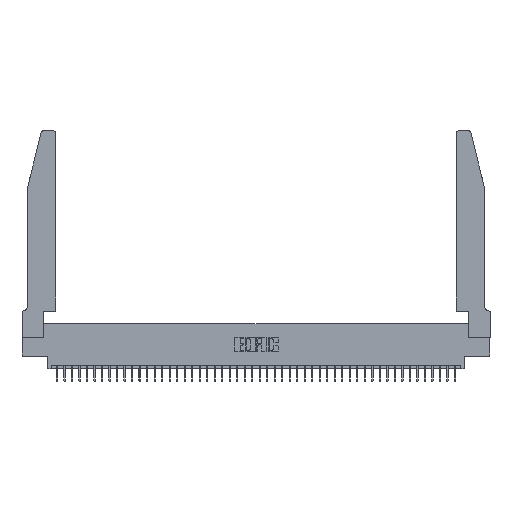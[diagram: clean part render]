
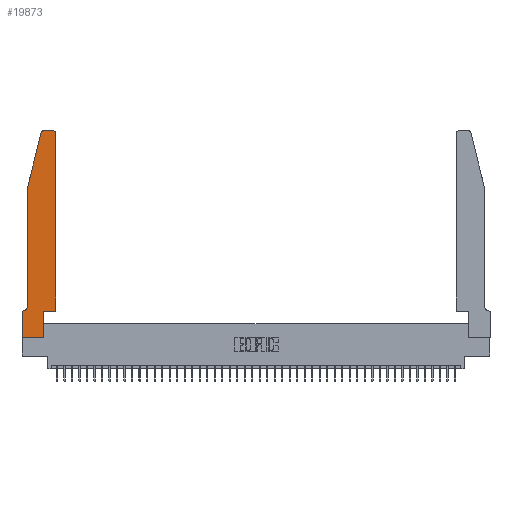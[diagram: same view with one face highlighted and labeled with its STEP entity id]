
A CAD part, top view. The second image highlights one B-rep face of the part: STEP entity #19873.
In plain terms, the highlighted planar face has unit normal (0, 0, 1).
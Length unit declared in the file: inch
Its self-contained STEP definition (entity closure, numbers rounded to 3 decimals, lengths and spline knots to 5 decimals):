
#1806 = CIRCLE ( 'NONE', #24319, 0.03 ) ;
#1857 = ORIENTED_EDGE ( 'NONE', *, *, #44088, .T. ) ;
#3058 = DIRECTION ( 'NONE',  ( 0., 1., 0. ) ) ;
#3879 = EDGE_CURVE ( 'NONE', #10807, #8634, #20952, .T. ) ;
#3942 = VERTEX_POINT ( 'NONE', #7230 ) ;
#4256 = ORIENTED_EDGE ( 'NONE', *, *, #16761, .T. ) ;
#4338 = DIRECTION ( 'NONE',  ( 0., 1., 0. ) ) ;
#4415 = AXIS2_PLACEMENT_3D ( 'NONE', #12191, #8808, #37184 ) ;
#4434 = CARTESIAN_POINT ( 'NONE',  ( 0.0755, 0.35, 0.37 ) ) ;
#4699 = EDGE_CURVE ( 'NONE', #20793, #45562, #8791, .T. ) ;
#4736 = CARTESIAN_POINT ( 'NONE',  ( 0., 0.35, 0.37 ) ) ;
#5658 = CARTESIAN_POINT ( 'NONE',  ( 0.0055, 0.42, 0.37 ) ) ;
#5793 = DIRECTION ( 'NONE',  ( 1., 0., 0. ) ) ;
#5996 = CARTESIAN_POINT ( 'NONE',  ( 0.2865, 0., 0.37 ) ) ;
#7230 = CARTESIAN_POINT ( 'NONE',  ( 0.284, 2.75, 0.37 ) ) ;
#7281 = LINE ( 'NONE', #4434, #15554 ) ;
#7769 = DIRECTION ( 'NONE',  ( 0., -1., 0. ) ) ;
#7910 = CARTESIAN_POINT ( 'NONE',  ( 0., 0., 0.37 ) ) ;
#8146 = ORIENTED_EDGE ( 'NONE', *, *, #43980, .T. ) ;
#8273 = DIRECTION ( 'NONE',  ( 1., 0., 0. ) ) ;
#8634 = VERTEX_POINT ( 'NONE', #21902 ) ;
#8762 = ORIENTED_EDGE ( 'NONE', *, *, #3879, .T. ) ;
#8791 = LINE ( 'NONE', #39439, #13723 ) ;
#8808 = DIRECTION ( 'NONE',  ( 0., 0., 1. ) ) ;
#9074 = CARTESIAN_POINT ( 'NONE',  ( 0., 0.35, 0.37 ) ) ;
#9474 = CIRCLE ( 'NONE', #20605, 0.07 ) ;
#10147 = ORIENTED_EDGE ( 'NONE', *, *, #39476, .T. ) ;
#10807 = VERTEX_POINT ( 'NONE', #34478 ) ;
#11122 = VECTOR ( 'NONE', #7769, 39.37008 ) ;
#11125 = EDGE_CURVE ( 'NONE', #25352, #10807, #15219, .T. ) ;
#11546 = DIRECTION ( 'NONE',  ( -1., 0., 0. ) ) ;
#11575 = LINE ( 'NONE', #18360, #22046 ) ;
#11656 = EDGE_LOOP ( 'NONE', ( #17000, #4256, #24188, #25541, #1857, #8146, #19244, #37994, #45067, #42346, #8762, #10147 ) ) ;
#12086 = DIRECTION ( 'NONE',  ( -1., 0., 0. ) ) ;
#12191 = CARTESIAN_POINT ( 'NONE',  ( 0.284, 2.72, 0.37 ) ) ;
#12465 = EDGE_CURVE ( 'NONE', #45123, #3942, #37187, .T. ) ;
#12601 = DIRECTION ( 'NONE',  ( 0., 0., 1. ) ) ;
#13723 = VECTOR ( 'NONE', #32603, 39.37008 ) ;
#13988 = LINE ( 'NONE', #44260, #25604 ) ;
#14217 = CARTESIAN_POINT ( 'NONE',  ( 0.4205, 2.75, 0.37 ) ) ;
#14949 = VECTOR ( 'NONE', #4338, 39.37008 ) ;
#15026 = CARTESIAN_POINT ( 'NONE',  ( 0.4505, 0.35, 0.37 ) ) ;
#15204 = DIRECTION ( 'NONE',  ( 0., 0., 1. ) ) ;
#15219 = LINE ( 'NONE', #15026, #20151 ) ;
#15293 = VERTEX_POINT ( 'NONE', #4736 ) ;
#15458 = EDGE_CURVE ( 'NONE', #15293, #20793, #13988, .T. ) ;
#15504 = AXIS2_PLACEMENT_3D ( 'NONE', #9074, #12601, #5793 ) ;
#15554 = VECTOR ( 'NONE', #11546, 39.37008 ) ;
#16761 = EDGE_CURVE ( 'NONE', #3942, #23194, #39832, .T. ) ;
#17000 = ORIENTED_EDGE ( 'NONE', *, *, #12465, .T. ) ;
#18360 = CARTESIAN_POINT ( 'NONE',  ( 0.0755, 2., 0.37 ) ) ;
#19244 = ORIENTED_EDGE ( 'NONE', *, *, #15458, .T. ) ;
#19538 = DIRECTION ( 'NONE',  ( 0., 0., -1. ) ) ;
#19554 = VERTEX_POINT ( 'NONE', #22153 ) ;
#19873 = ADVANCED_FACE ( 'NONE', ( #30736 ), #26960, .T. ) ;
#20133 = DIRECTION ( 'NONE',  ( 0., -1., 0. ) ) ;
#20151 = VECTOR ( 'NONE', #36160, 39.37008 ) ;
#20487 = CARTESIAN_POINT ( 'NONE',  ( 0.4505, 0.35, 0.37 ) ) ;
#20605 = AXIS2_PLACEMENT_3D ( 'NONE', #5658, #19538, #34046 ) ;
#20793 = VERTEX_POINT ( 'NONE', #7910 ) ;
#20952 = LINE ( 'NONE', #20487, #39786 ) ;
#21011 = CARTESIAN_POINT ( 'NONE',  ( 0.0755, 2., 0.37 ) ) ;
#21902 = CARTESIAN_POINT ( 'NONE',  ( 0.4505, 2.72, 0.37 ) ) ;
#22046 = VECTOR ( 'NONE', #43245, 39.37008 ) ;
#22153 = CARTESIAN_POINT ( 'NONE',  ( 0.0755, 0.42, 0.37 ) ) ;
#23194 = VERTEX_POINT ( 'NONE', #42938 ) ;
#24188 = ORIENTED_EDGE ( 'NONE', *, *, #45297, .T. ) ;
#24250 = VERTEX_POINT ( 'NONE', #21011 ) ;
#24319 = AXIS2_PLACEMENT_3D ( 'NONE', #25851, #15204, #8273 ) ;
#25352 = VERTEX_POINT ( 'NONE', #37000 ) ;
#25541 = ORIENTED_EDGE ( 'NONE', *, *, #43533, .T. ) ;
#25594 = VECTOR ( 'NONE', #12086, 39.37008 ) ;
#25604 = VECTOR ( 'NONE', #20133, 39.37008 ) ;
#25663 = CARTESIAN_POINT ( 'NONE',  ( 0.0755, 2., 0.37 ) ) ;
#25851 = CARTESIAN_POINT ( 'NONE',  ( 0.4205, 2.72, 0.37 ) ) ;
#26960 = PLANE ( 'NONE',  #15504 ) ;
#29878 = LINE ( 'NONE', #25663, #11122 ) ;
#30736 = FACE_OUTER_BOUND ( 'NONE', #11656, .T. ) ;
#32603 = DIRECTION ( 'NONE',  ( 1., 0., 0. ) ) ;
#34046 = DIRECTION ( 'NONE',  ( -1., 0., 0. ) ) ;
#34478 = CARTESIAN_POINT ( 'NONE',  ( 0.4505, 0.35, 0.37 ) ) ;
#35109 = EDGE_CURVE ( 'NONE', #45562, #25352, #43716, .T. ) ;
#36160 = DIRECTION ( 'NONE',  ( 1., 0., 0. ) ) ;
#36313 = CARTESIAN_POINT ( 'NONE',  ( 0.2605, 2.75, 0.37 ) ) ;
#37000 = CARTESIAN_POINT ( 'NONE',  ( 0.2865, 0.35, 0.37 ) ) ;
#37184 = DIRECTION ( 'NONE',  ( 1., 0., 0. ) ) ;
#37187 = LINE ( 'NONE', #36313, #25594 ) ;
#37994 = ORIENTED_EDGE ( 'NONE', *, *, #4699, .T. ) ;
#38793 = CARTESIAN_POINT ( 'NONE',  ( 0.0055, 0.35, 0.37 ) ) ;
#39439 = CARTESIAN_POINT ( 'NONE',  ( 0., 0., 0.37 ) ) ;
#39476 = EDGE_CURVE ( 'NONE', #8634, #45123, #1806, .T. ) ;
#39786 = VECTOR ( 'NONE', #3058, 39.37008 ) ;
#39832 = CIRCLE ( 'NONE', #4415, 0.03 ) ;
#41490 = VERTEX_POINT ( 'NONE', #38793 ) ;
#42346 = ORIENTED_EDGE ( 'NONE', *, *, #11125, .T. ) ;
#42938 = CARTESIAN_POINT ( 'NONE',  ( 0.25487, 2.72718, 0.37 ) ) ;
#43245 = DIRECTION ( 'NONE',  ( -0.239, -0.971, 0. ) ) ;
#43413 = CARTESIAN_POINT ( 'NONE',  ( 0.2865, 0.35, 0.37 ) ) ;
#43533 = EDGE_CURVE ( 'NONE', #24250, #19554, #29878, .T. ) ;
#43716 = LINE ( 'NONE', #43413, #14949 ) ;
#43980 = EDGE_CURVE ( 'NONE', #41490, #15293, #7281, .T. ) ;
#44088 = EDGE_CURVE ( 'NONE', #19554, #41490, #9474, .T. ) ;
#44260 = CARTESIAN_POINT ( 'NONE',  ( 0., 0., 0.37 ) ) ;
#45067 = ORIENTED_EDGE ( 'NONE', *, *, #35109, .T. ) ;
#45123 = VERTEX_POINT ( 'NONE', #14217 ) ;
#45297 = EDGE_CURVE ( 'NONE', #23194, #24250, #11575, .T. ) ;
#45562 = VERTEX_POINT ( 'NONE', #5996 ) ;
